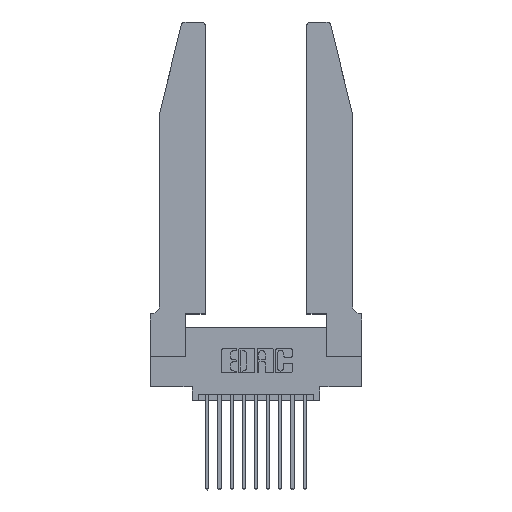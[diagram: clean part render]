
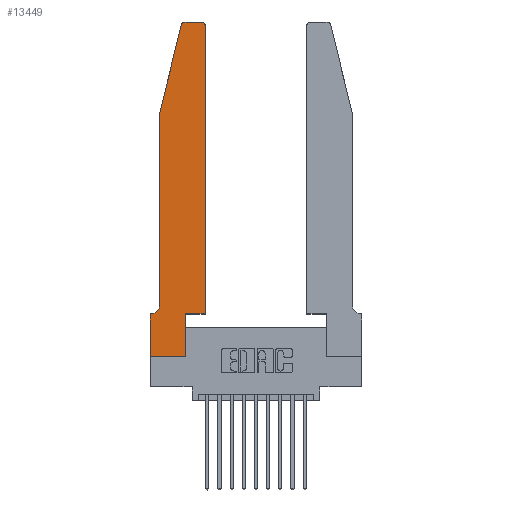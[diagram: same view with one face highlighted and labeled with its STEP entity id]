
A CAD part, top view. The second image highlights one B-rep face of the part: STEP entity #13449.
In plain terms, the highlighted planar face has unit normal (0, 0, 1).
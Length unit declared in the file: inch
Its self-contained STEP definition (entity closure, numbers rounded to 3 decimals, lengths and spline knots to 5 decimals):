
#248 = VERTEX_POINT ( 'NONE', #1826 ) ;
#268 = VERTEX_POINT ( 'NONE', #15804 ) ;
#433 = ORIENTED_EDGE ( 'NONE', *, *, #12921, .T. ) ;
#492 = PLANE ( 'NONE',  #4605 ) ;
#541 = CARTESIAN_POINT ( 'NONE',  ( 0.4205, 2.75, 0.37 ) ) ;
#545 = CARTESIAN_POINT ( 'NONE',  ( 0., 0.35, 0.37 ) ) ;
#1026 = VERTEX_POINT ( 'NONE', #541 ) ;
#1124 = CIRCLE ( 'NONE', #4439, 0.07 ) ;
#1226 = VECTOR ( 'NONE', #14485, 39.37008 ) ;
#1230 = FACE_OUTER_BOUND ( 'NONE', #6564, .T. ) ;
#1231 = AXIS2_PLACEMENT_3D ( 'NONE', #10492, #5361, #1550 ) ;
#1326 = CIRCLE ( 'NONE', #14309, 0.03 ) ;
#1550 = DIRECTION ( 'NONE',  ( 1., 0., 0. ) ) ;
#1645 = DIRECTION ( 'NONE',  ( 1., 0., 0. ) ) ;
#1698 = CARTESIAN_POINT ( 'NONE',  ( 0.0755, 0.42, 0.37 ) ) ;
#1762 = CARTESIAN_POINT ( 'NONE',  ( 0.25487, 2.72718, 0.37 ) ) ;
#1826 = CARTESIAN_POINT ( 'NONE',  ( 0.2865, 0., 0.37 ) ) ;
#1827 = VECTOR ( 'NONE', #5252, 39.37008 ) ;
#1862 = VERTEX_POINT ( 'NONE', #3563 ) ;
#1917 = DIRECTION ( 'NONE',  ( 0., 0., 1. ) ) ;
#1968 = EDGE_CURVE ( 'NONE', #10268, #11138, #1326, .T. ) ;
#2075 = ORIENTED_EDGE ( 'NONE', *, *, #4902, .T. ) ;
#2295 = VERTEX_POINT ( 'NONE', #10901 ) ;
#2329 = VECTOR ( 'NONE', #13395, 39.37008 ) ;
#2409 = VERTEX_POINT ( 'NONE', #1698 ) ;
#2425 = ORIENTED_EDGE ( 'NONE', *, *, #5108, .T. ) ;
#2798 = CARTESIAN_POINT ( 'NONE',  ( 0.0755, 2., 0.37 ) ) ;
#2923 = ORIENTED_EDGE ( 'NONE', *, *, #3480, .T. ) ;
#3330 = LINE ( 'NONE', #13079, #7695 ) ;
#3480 = EDGE_CURVE ( 'NONE', #5662, #2409, #5441, .T. ) ;
#3537 = CARTESIAN_POINT ( 'NONE',  ( 0.0755, 2., 0.37 ) ) ;
#3563 = CARTESIAN_POINT ( 'NONE',  ( 0.4505, 0.35, 0.37 ) ) ;
#4016 = CARTESIAN_POINT ( 'NONE',  ( 0.0055, 0.35, 0.37 ) ) ;
#4157 = VECTOR ( 'NONE', #7288, 39.37008 ) ;
#4163 = ORIENTED_EDGE ( 'NONE', *, *, #5701, .T. ) ;
#4246 = CARTESIAN_POINT ( 'NONE',  ( 0., 0., 0.37 ) ) ;
#4300 = ORIENTED_EDGE ( 'NONE', *, *, #12473, .T. ) ;
#4327 = VERTEX_POINT ( 'NONE', #4016 ) ;
#4362 = VECTOR ( 'NONE', #15357, 39.37008 ) ;
#4439 = AXIS2_PLACEMENT_3D ( 'NONE', #12893, #8100, #13404 ) ;
#4605 = AXIS2_PLACEMENT_3D ( 'NONE', #11974, #1917, #14633 ) ;
#4692 = DIRECTION ( 'NONE',  ( 0., 0., 1. ) ) ;
#4902 = EDGE_CURVE ( 'NONE', #248, #2295, #11382, .T. ) ;
#5108 = EDGE_CURVE ( 'NONE', #11893, #1026, #15733, .T. ) ;
#5252 = DIRECTION ( 'NONE',  ( -1., 0., 0. ) ) ;
#5361 = DIRECTION ( 'NONE',  ( 0., 0., 1. ) ) ;
#5441 = LINE ( 'NONE', #2798, #8631 ) ;
#5662 = VERTEX_POINT ( 'NONE', #7117 ) ;
#5701 = EDGE_CURVE ( 'NONE', #2409, #4327, #1124, .T. ) ;
#6172 = CARTESIAN_POINT ( 'NONE',  ( 0.284, 2.72, 0.37 ) ) ;
#6198 = ORIENTED_EDGE ( 'NONE', *, *, #10912, .T. ) ;
#6310 = CARTESIAN_POINT ( 'NONE',  ( 0.2605, 2.75, 0.37 ) ) ;
#6564 = EDGE_LOOP ( 'NONE', ( #8474, #8245, #6198, #2923, #4163, #15917, #4300, #14156, #2075, #433, #12013, #2425 ) ) ;
#6831 = DIRECTION ( 'NONE',  ( -1., 0., 0. ) ) ;
#7117 = CARTESIAN_POINT ( 'NONE',  ( 0.0755, 2., 0.37 ) ) ;
#7288 = DIRECTION ( 'NONE',  ( 0., 1., 0. ) ) ;
#7370 = LINE ( 'NONE', #4246, #1226 ) ;
#7695 = VECTOR ( 'NONE', #6831, 39.37008 ) ;
#8036 = DIRECTION ( 'NONE',  ( 0., 1., 0. ) ) ;
#8100 = DIRECTION ( 'NONE',  ( 0., 0., -1. ) ) ;
#8245 = ORIENTED_EDGE ( 'NONE', *, *, #1968, .T. ) ;
#8474 = ORIENTED_EDGE ( 'NONE', *, *, #13787, .T. ) ;
#8565 = DIRECTION ( 'NONE',  ( 1., 0., 0. ) ) ;
#8631 = VECTOR ( 'NONE', #11687, 39.37008 ) ;
#9382 = LINE ( 'NONE', #14252, #11381 ) ;
#9877 = LINE ( 'NONE', #14818, #2329 ) ;
#9879 = EDGE_CURVE ( 'NONE', #268, #248, #7370, .T. ) ;
#10167 = CARTESIAN_POINT ( 'NONE',  ( 0.2865, 0.35, 0.37 ) ) ;
#10268 = VERTEX_POINT ( 'NONE', #11498 ) ;
#10492 = CARTESIAN_POINT ( 'NONE',  ( 0.4205, 2.72, 0.37 ) ) ;
#10901 = CARTESIAN_POINT ( 'NONE',  ( 0.2865, 0.35, 0.37 ) ) ;
#10912 = EDGE_CURVE ( 'NONE', #11138, #5662, #16096, .T. ) ;
#11138 = VERTEX_POINT ( 'NONE', #1762 ) ;
#11381 = VECTOR ( 'NONE', #1645, 39.37008 ) ;
#11382 = LINE ( 'NONE', #10167, #14560 ) ;
#11498 = CARTESIAN_POINT ( 'NONE',  ( 0.284, 2.75, 0.37 ) ) ;
#11687 = DIRECTION ( 'NONE',  ( 0., -1., 0. ) ) ;
#11753 = EDGE_CURVE ( 'NONE', #4327, #11754, #3330, .T. ) ;
#11754 = VERTEX_POINT ( 'NONE', #545 ) ;
#11893 = VERTEX_POINT ( 'NONE', #16001 ) ;
#11974 = CARTESIAN_POINT ( 'NONE',  ( 0., 0.35, 0.37 ) ) ;
#12013 = ORIENTED_EDGE ( 'NONE', *, *, #14702, .T. ) ;
#12473 = EDGE_CURVE ( 'NONE', #11754, #268, #9877, .T. ) ;
#12893 = CARTESIAN_POINT ( 'NONE',  ( 0.0055, 0.42, 0.37 ) ) ;
#12921 = EDGE_CURVE ( 'NONE', #2295, #1862, #9382, .T. ) ;
#13079 = CARTESIAN_POINT ( 'NONE',  ( 0.0755, 0.35, 0.37 ) ) ;
#13395 = DIRECTION ( 'NONE',  ( 0., -1., 0. ) ) ;
#13404 = DIRECTION ( 'NONE',  ( -1., 0., 0. ) ) ;
#13449 = ADVANCED_FACE ( 'NONE', ( #1230 ), #492, .T. ) ;
#13762 = LINE ( 'NONE', #6310, #1827 ) ;
#13787 = EDGE_CURVE ( 'NONE', #1026, #10268, #13762, .T. ) ;
#14156 = ORIENTED_EDGE ( 'NONE', *, *, #9879, .T. ) ;
#14252 = CARTESIAN_POINT ( 'NONE',  ( 0.4505, 0.35, 0.37 ) ) ;
#14309 = AXIS2_PLACEMENT_3D ( 'NONE', #6172, #4692, #8565 ) ;
#14485 = DIRECTION ( 'NONE',  ( 1., 0., 0. ) ) ;
#14560 = VECTOR ( 'NONE', #8036, 39.37008 ) ;
#14633 = DIRECTION ( 'NONE',  ( 1., 0., 0. ) ) ;
#14702 = EDGE_CURVE ( 'NONE', #1862, #11893, #15479, .T. ) ;
#14818 = CARTESIAN_POINT ( 'NONE',  ( 0., 0., 0.37 ) ) ;
#14902 = CARTESIAN_POINT ( 'NONE',  ( 0.4505, 0.35, 0.37 ) ) ;
#15357 = DIRECTION ( 'NONE',  ( -0.239, -0.971, 0. ) ) ;
#15479 = LINE ( 'NONE', #14902, #4157 ) ;
#15733 = CIRCLE ( 'NONE', #1231, 0.03 ) ;
#15804 = CARTESIAN_POINT ( 'NONE',  ( 0., 0., 0.37 ) ) ;
#15917 = ORIENTED_EDGE ( 'NONE', *, *, #11753, .T. ) ;
#16001 = CARTESIAN_POINT ( 'NONE',  ( 0.4505, 2.72, 0.37 ) ) ;
#16096 = LINE ( 'NONE', #3537, #4362 ) ;
